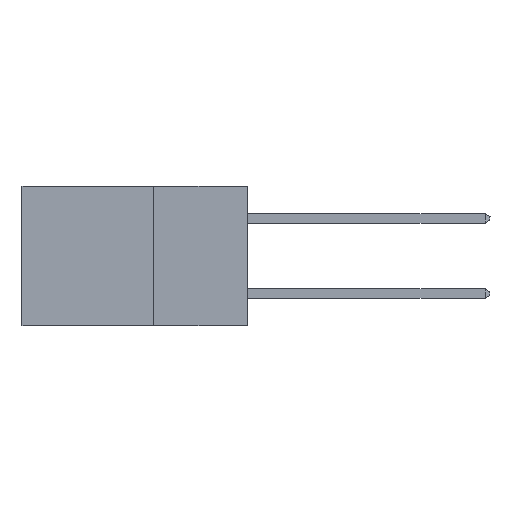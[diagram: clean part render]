
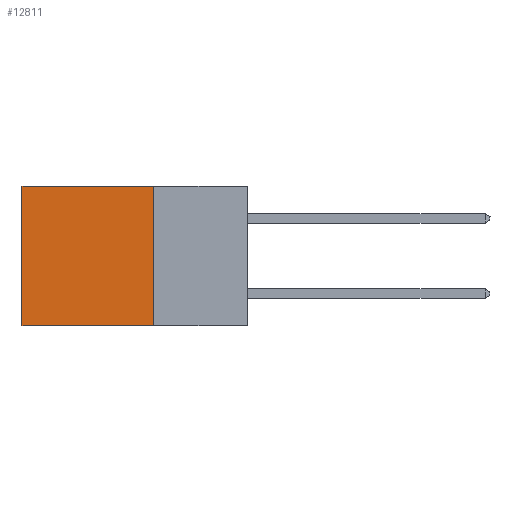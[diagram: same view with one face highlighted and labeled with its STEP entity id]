
A CAD part, left-side view. The second image highlights one B-rep face of the part: STEP entity #12811.
In plain terms, the highlighted planar face has unit normal (-1, 0, 0).
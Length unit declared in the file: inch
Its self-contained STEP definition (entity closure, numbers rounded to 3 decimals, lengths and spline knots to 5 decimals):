
#192 = DIRECTION ( 'NONE',  ( 0., 0., -1. ) ) ;
#225 = EDGE_LOOP ( 'NONE', ( #13047, #12592, #5816, #11847 ) ) ;
#473 = LINE ( 'NONE', #13721, #8927 ) ;
#772 = VERTEX_POINT ( 'NONE', #12048 ) ;
#822 = DIRECTION ( 'NONE',  ( 0., 1., 0. ) ) ;
#2102 = CARTESIAN_POINT ( 'NONE',  ( 0.298, 0.6, 0. ) ) ;
#2872 = VECTOR ( 'NONE', #13064, 39.37008 ) ;
#2902 = VERTEX_POINT ( 'NONE', #12121 ) ;
#3130 = CARTESIAN_POINT ( 'NONE',  ( 0.298, 0.25, 0. ) ) ;
#3243 = VERTEX_POINT ( 'NONE', #2102 ) ;
#3436 = CARTESIAN_POINT ( 'NONE',  ( 0.298, 0.25, -0.37 ) ) ;
#3435 = VECTOR ( 'NONE', #12745, 39.37008 ) ;
#5482 = EDGE_CURVE ( 'NONE', #8221, #772, #473, .T. ) ;
#5816 = ORIENTED_EDGE ( 'NONE', *, *, #5482, .F. ) ;
#6911 = DIRECTION ( 'NONE',  ( 1., 0., 0. ) ) ;
#7926 = EDGE_CURVE ( 'NONE', #772, #2902, #11494, .T. ) ;
#8146 = AXIS2_PLACEMENT_3D ( 'NONE', #3130, #6911, #14239 ) ;
#8221 = VERTEX_POINT ( 'NONE', #15701 ) ;
#8267 = CARTESIAN_POINT ( 'NONE',  ( 0.298, 0.6, 0. ) ) ;
#8427 = LINE ( 'NONE', #8267, #3435 ) ;
#8927 = VECTOR ( 'NONE', #192, 39.37008 ) ;
#9261 = EDGE_CURVE ( 'NONE', #3243, #2902, #8427, .T. ) ;
#9325 = EDGE_CURVE ( 'NONE', #8221, #3243, #12015, .T. ) ;
#10309 = CARTESIAN_POINT ( 'NONE',  ( 0.298, 0.25, 0. ) ) ;
#11494 = LINE ( 'NONE', #3436, #2872 ) ;
#11735 = PLANE ( 'NONE',  #8146 ) ;
#11847 = ORIENTED_EDGE ( 'NONE', *, *, #9325, .T. ) ;
#12015 = LINE ( 'NONE', #10309, #13573 ) ;
#12048 = CARTESIAN_POINT ( 'NONE',  ( 0.298, 0.25, -0.37 ) ) ;
#12121 = CARTESIAN_POINT ( 'NONE',  ( 0.298, 0.6, -0.37 ) ) ;
#12592 = ORIENTED_EDGE ( 'NONE', *, *, #7926, .F. ) ;
#12745 = DIRECTION ( 'NONE',  ( 0., 0., -1. ) ) ;
#12811 = ADVANCED_FACE ( 'NONE', ( #15035 ), #11735, .F. ) ;
#13047 = ORIENTED_EDGE ( 'NONE', *, *, #9261, .T. ) ;
#13064 = DIRECTION ( 'NONE',  ( 0., 1., 0. ) ) ;
#13573 = VECTOR ( 'NONE', #822, 39.37008 ) ;
#13721 = CARTESIAN_POINT ( 'NONE',  ( 0.298, 0.25, 0. ) ) ;
#14239 = DIRECTION ( 'NONE',  ( 0., 0., -1. ) ) ;
#15035 = FACE_OUTER_BOUND ( 'NONE', #225, .T. ) ;
#15701 = CARTESIAN_POINT ( 'NONE',  ( 0.298, 0.25, 0. ) ) ;
